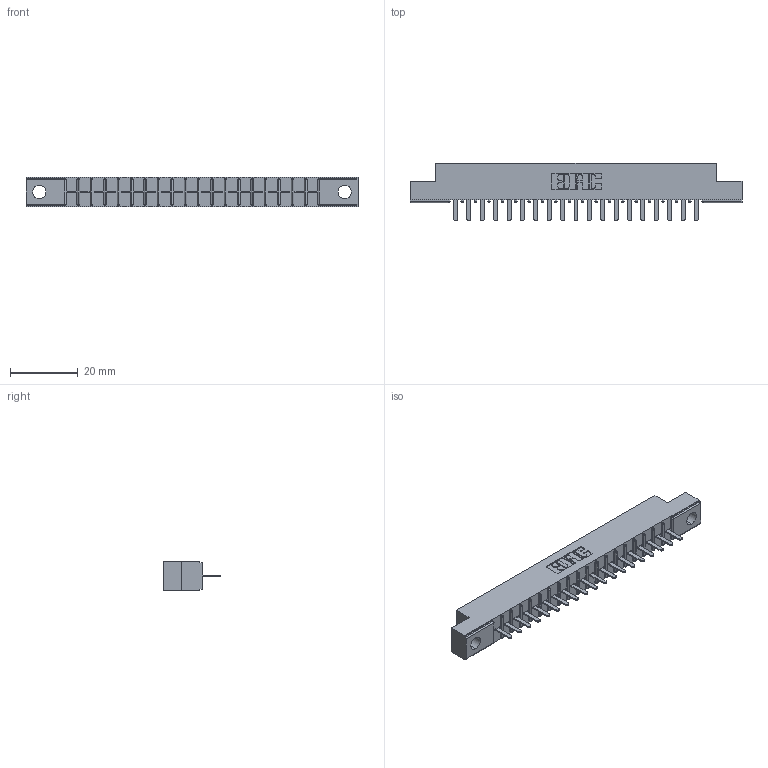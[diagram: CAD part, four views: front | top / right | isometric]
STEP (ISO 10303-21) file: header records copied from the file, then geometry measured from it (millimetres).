
FILE_DESCRIPTION (( 'STEP AP203' ), '1' );
FILE_NAME ('356-019-520-104.STEP', '2018-08-01T19:35:39', ( '' ), ( '' ), 'SwSTEP 2.0', 'SolidWorks 2016', '' );
FILE_SCHEMA (( 'CONFIG_CONTROL_DESIGN' ));
Length unit declared in the file: inch
Products named in the file (3): 306 Part_.156 Dia; 306-290-001_120; 356-019-520-104
Assembly tree (20 placements, depth 2):
  356-019-520-104
    306 Part_.156 Dia
    306-290-001_120  x19
Bounding box: 98.3 x 17.12 x 8.71 mm (x, y, z)
Volume: 6602.4 mm3; surface area: 9541.6 mm2
Topology: 20 solids, 20 shells, 1460 faces, 4095 edges, 2626 vertices
Faces by surface type: plane 975, cylinder 409, sphere 76
Entity records: 21072 total; most frequent: CARTESIAN_POINT 3538, ORIENTED_EDGE 3502, DIRECTION 3483, EDGE_CURVE 1751, VECTOR 1365, LINE 1365, VERTEX_POINT 1114, AXIS2_PLACEMENT_3D 1059
